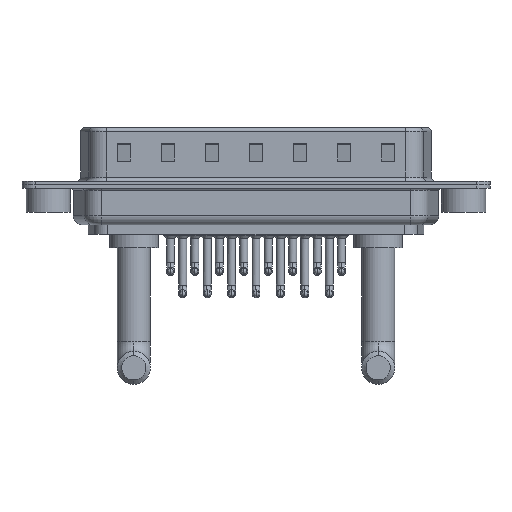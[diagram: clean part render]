
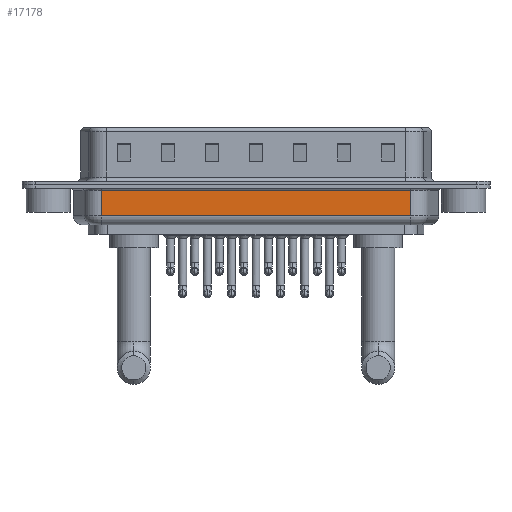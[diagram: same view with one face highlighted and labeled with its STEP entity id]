
A CAD part, front view. The second image highlights one B-rep face of the part: STEP entity #17178.
In plain terms, the highlighted planar face has unit normal (0, -1, 0).
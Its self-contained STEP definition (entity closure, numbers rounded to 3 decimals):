
#681 = CARTESIAN_POINT ( 'NONE',  ( 6.006, -5.35, -4.5 ) ) ;
#838 = CARTESIAN_POINT ( 'NONE',  ( 41.044, -5.35, -0.65 ) ) ;
#1680 = EDGE_CURVE ( 'NONE', #21541, #6831, #8957, .T. ) ;
#1940 = VECTOR ( 'NONE', #21101, 1000. ) ;
#3766 = EDGE_LOOP ( 'NONE', ( #17256, #19749, #23934, #22016 ) ) ;
#4448 = FACE_OUTER_BOUND ( 'NONE', #3766, .T. ) ;
#4925 = CARTESIAN_POINT ( 'NONE',  ( 41.044, -5.35, -4.5 ) ) ;
#5086 = CARTESIAN_POINT ( 'NONE',  ( 41.044, -5.35, -3.5 ) ) ;
#6059 = LINE ( 'NONE', #7708, #1940 ) ;
#6315 = EDGE_CURVE ( 'NONE', #8812, #13114, #8066, .T. ) ;
#6808 = DIRECTION ( 'NONE',  ( 0., 0., 1. ) ) ;
#6831 = VERTEX_POINT ( 'NONE', #838 ) ;
#7285 = VECTOR ( 'NONE', #6808, 1000. ) ;
#7543 = EDGE_CURVE ( 'NONE', #8812, #21541, #6059, .T. ) ;
#7708 = CARTESIAN_POINT ( 'NONE',  ( 6.006, -5.35, -3.5 ) ) ;
#8066 = LINE ( 'NONE', #15351, #13931 ) ;
#8812 = VERTEX_POINT ( 'NONE', #16069 ) ;
#8957 = LINE ( 'NONE', #4925, #7285 ) ;
#9833 = LINE ( 'NONE', #23222, #11620 ) ;
#11620 = VECTOR ( 'NONE', #13706, 1000. ) ;
#11975 = DIRECTION ( 'NONE',  ( 0., 0., 1. ) ) ;
#12098 = PLANE ( 'NONE',  #12529 ) ;
#12529 = AXIS2_PLACEMENT_3D ( 'NONE', #681, #17488, #11975 ) ;
#12621 = EDGE_CURVE ( 'NONE', #6831, #13114, #9833, .T. ) ;
#13114 = VERTEX_POINT ( 'NONE', #20755 ) ;
#13592 = DIRECTION ( 'NONE',  ( 0., 0., 1. ) ) ;
#13706 = DIRECTION ( 'NONE',  ( -1., 0., 0. ) ) ;
#13931 = VECTOR ( 'NONE', #13592, 1000. ) ;
#15351 = CARTESIAN_POINT ( 'NONE',  ( 6.006, -5.35, -4.5 ) ) ;
#16069 = CARTESIAN_POINT ( 'NONE',  ( 6.006, -5.35, -3.5 ) ) ;
#17178 = ADVANCED_FACE ( 'NONE', ( #4448 ), #12098, .F. ) ;
#17256 = ORIENTED_EDGE ( 'NONE', *, *, #6315, .F. ) ;
#17488 = DIRECTION ( 'NONE',  ( 0., 1., 0. ) ) ;
#19749 = ORIENTED_EDGE ( 'NONE', *, *, #7543, .T. ) ;
#20755 = CARTESIAN_POINT ( 'NONE',  ( 6.006, -5.35, -0.65 ) ) ;
#21101 = DIRECTION ( 'NONE',  ( 1., 0., 0. ) ) ;
#21541 = VERTEX_POINT ( 'NONE', #5086 ) ;
#22016 = ORIENTED_EDGE ( 'NONE', *, *, #12621, .T. ) ;
#23222 = CARTESIAN_POINT ( 'NONE',  ( 6.006, -5.35, -0.65 ) ) ;
#23934 = ORIENTED_EDGE ( 'NONE', *, *, #1680, .T. ) ;
